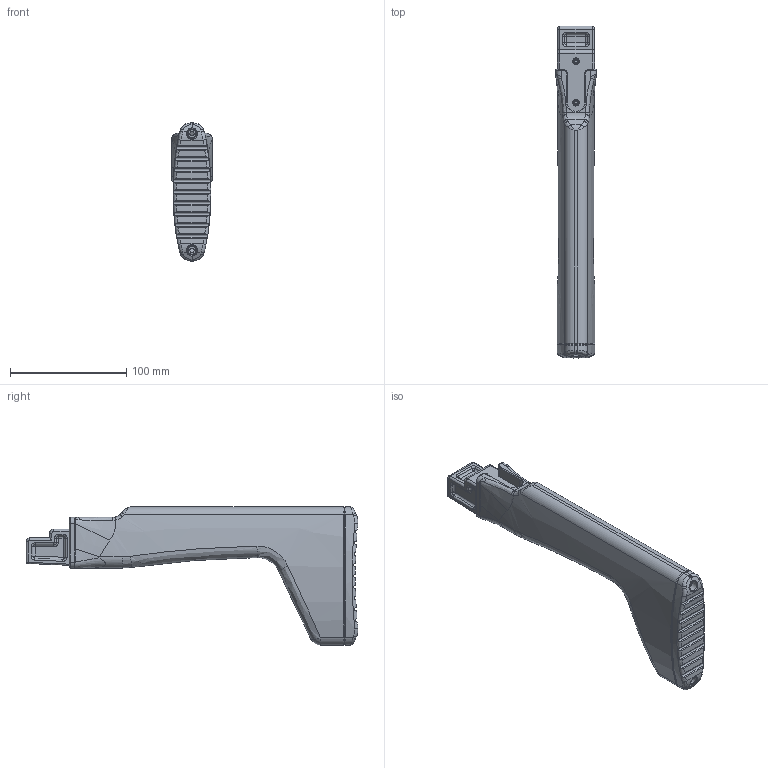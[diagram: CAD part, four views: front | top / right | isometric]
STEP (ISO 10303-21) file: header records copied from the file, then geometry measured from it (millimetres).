
FILE_DESCRIPTION(/* description */ (''),/* implementation_level */ '2;1');
FILE_NAME(/* name */ 'Single Piece Stock.step',/* time_stamp */ '2021-10-03T06:59:41-04:00',/* author */ (''),/* organization */ (''),/* preprocessor_version */ 'ST-DEVELOPER v18.1',/* originating_system */ 'Autodesk Translation Framework v10.10.0.1391',/* authorisation */ '');
FILE_SCHEMA (('AUTOMOTIVE_DESIGN { 1 0 10303 214 3 1 1 }'));
Length unit declared in the file: millimetre
Products named in the file (1): Full Stock
Bounding box: 35 x 285.01 x 118.61 mm (x, y, z)
Volume: 256494.5 mm3; surface area: 83438.6 mm2
Topology: 2 solids, 2 shells, 567 faces, 1307 edges, 755 vertices
Faces by surface type: bspline 239, cylinder 177, plane 60, torus 49, sphere 30, cone 12
Full cylindrical faces by diameter (mm): 2.636 x2, 3.8 x4, 4.6 x2, 8 x2
Entity records: 24165 total; most frequent: CARTESIAN_POINT 12641, ORIENTED_EDGE 2598, DIRECTION 2021, EDGE_CURVE 1299, AXIS2_PLACEMENT_3D 835, VERTEX_POINT 755, EDGE_LOOP 594, FACE_OUTER_BOUND 567
